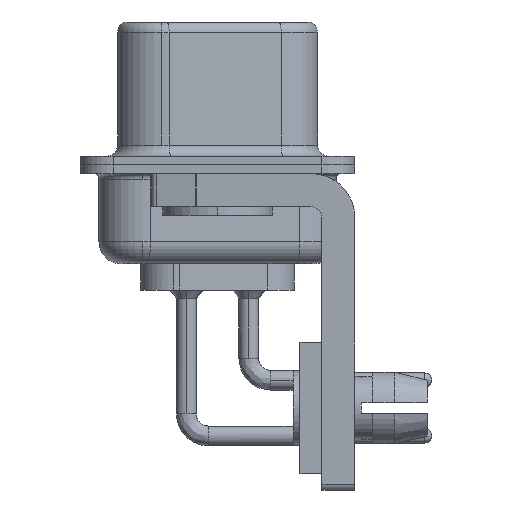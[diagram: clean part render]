
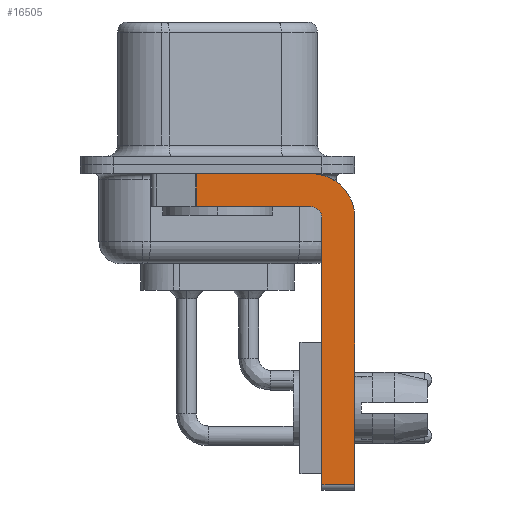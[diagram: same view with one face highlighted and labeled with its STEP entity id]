
A CAD part, left-side view. The second image highlights one B-rep face of the part: STEP entity #16505.
In plain terms, the highlighted planar face has unit normal (-1, 0, 0).
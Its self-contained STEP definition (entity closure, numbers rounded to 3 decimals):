
#245 = EDGE_CURVE ( 'NONE', #12847, #6155, #29911, .T. ) ;
#1064 = CARTESIAN_POINT ( 'NONE',  ( -2.9, -4.25, -2.4 ) ) ;
#1398 = DIRECTION ( 'NONE',  ( 1., 0., 0. ) ) ;
#1593 = ORIENTED_EDGE ( 'NONE', *, *, #245, .F. ) ;
#1625 = VECTOR ( 'NONE', #12792, 1000. ) ;
#1998 = LINE ( 'NONE', #26035, #20230 ) ;
#2313 = DIRECTION ( 'NONE',  ( 0., 0., -1. ) ) ;
#2340 = DIRECTION ( 'NONE',  ( 1., 0., 0. ) ) ;
#2969 = ORIENTED_EDGE ( 'NONE', *, *, #7836, .F. ) ;
#2994 = CARTESIAN_POINT ( 'NONE',  ( -2.9, 3., -0.4 ) ) ;
#3053 = CARTESIAN_POINT ( 'NONE',  ( -2.9, -4.75, -14.55 ) ) ;
#3404 = DIRECTION ( 'NONE',  ( 0., 0., 1. ) ) ;
#3484 = EDGE_LOOP ( 'NONE', ( #2969, #8541, #24831, #27332, #15916, #27538, #18704, #1593 ) ) ;
#3966 = VERTEX_POINT ( 'NONE', #19631 ) ;
#4508 = CARTESIAN_POINT ( 'NONE',  ( -2.9, -4.25, -1.9 ) ) ;
#4924 = VERTEX_POINT ( 'NONE', #22177 ) ;
#5443 = DIRECTION ( 'NONE',  ( 0., -1., 0. ) ) ;
#5707 = CARTESIAN_POINT ( 'NONE',  ( -2.9, 0.978, -1.9 ) ) ;
#6155 = VERTEX_POINT ( 'NONE', #12769 ) ;
#7708 = LINE ( 'NONE', #5707, #1625 ) ;
#7836 = EDGE_CURVE ( 'NONE', #9956, #12847, #29578, .T. ) ;
#7934 = EDGE_CURVE ( 'NONE', #3966, #4924, #8753, .T. ) ;
#8349 = CARTESIAN_POINT ( 'NONE',  ( -2.9, -4.25, -0.4 ) ) ;
#8541 = ORIENTED_EDGE ( 'NONE', *, *, #23324, .T. ) ;
#8753 = CIRCLE ( 'NONE', #9552, 0.5 ) ;
#9113 = DIRECTION ( 'NONE',  ( 0., 1., 0. ) ) ;
#9251 = DIRECTION ( 'NONE',  ( 0., 0., 1. ) ) ;
#9552 = AXIS2_PLACEMENT_3D ( 'NONE', #1064, #17651, #3404 ) ;
#9956 = VERTEX_POINT ( 'NONE', #14706 ) ;
#10140 = AXIS2_PLACEMENT_3D ( 'NONE', #15537, #1398, #17988 ) ;
#10215 = CARTESIAN_POINT ( 'NONE',  ( -2.9, -6.25, -14.55 ) ) ;
#10776 = VERTEX_POINT ( 'NONE', #10215 ) ;
#10847 = LINE ( 'NONE', #4508, #22965 ) ;
#11173 = CARTESIAN_POINT ( 'NONE',  ( -2.9, -6.25, -2.4 ) ) ;
#12101 = VECTOR ( 'NONE', #5443, 1000. ) ;
#12769 = CARTESIAN_POINT ( 'NONE',  ( -2.9, -6.25, -2.4 ) ) ;
#12792 = DIRECTION ( 'NONE',  ( 0., 0., -1. ) ) ;
#12847 = VERTEX_POINT ( 'NONE', #8349 ) ;
#13667 = VERTEX_POINT ( 'NONE', #3053 ) ;
#13710 = EDGE_CURVE ( 'NONE', #13667, #10776, #28885, .T. ) ;
#13992 = FACE_OUTER_BOUND ( 'NONE', #3484, .T. ) ;
#14706 = CARTESIAN_POINT ( 'NONE',  ( -2.9, 0.978, -0.4 ) ) ;
#14728 = DIRECTION ( 'NONE',  ( 0., -1., 0. ) ) ;
#15537 = CARTESIAN_POINT ( 'NONE',  ( -2.9, -4.25, -2.4 ) ) ;
#15916 = ORIENTED_EDGE ( 'NONE', *, *, #28440, .F. ) ;
#16208 = EDGE_CURVE ( 'NONE', #4924, #29342, #10847, .T. ) ;
#16505 = ADVANCED_FACE ( 'NONE', ( #13992 ), #24970, .F. ) ;
#16553 = AXIS2_PLACEMENT_3D ( 'NONE', #18113, #2340, #2313 ) ;
#16686 = EDGE_CURVE ( 'NONE', #6155, #10776, #28485, .T. ) ;
#17651 = DIRECTION ( 'NONE',  ( -1., 0., 0. ) ) ;
#17988 = DIRECTION ( 'NONE',  ( 0., 0., -1. ) ) ;
#18113 = CARTESIAN_POINT ( 'NONE',  ( -2.9, -4.25, -2.4 ) ) ;
#18704 = ORIENTED_EDGE ( 'NONE', *, *, #16686, .F. ) ;
#19631 = CARTESIAN_POINT ( 'NONE',  ( -2.9, -4.75, -2.4 ) ) ;
#19819 = CARTESIAN_POINT ( 'NONE',  ( -2.9, -4.25, -14.55 ) ) ;
#20230 = VECTOR ( 'NONE', #9251, 1000. ) ;
#20277 = CARTESIAN_POINT ( 'NONE',  ( -2.9, 0.978, -1.9 ) ) ;
#22177 = CARTESIAN_POINT ( 'NONE',  ( -2.9, -4.25, -1.9 ) ) ;
#22686 = VECTOR ( 'NONE', #14728, 1000. ) ;
#22965 = VECTOR ( 'NONE', #9113, 1000. ) ;
#23067 = VECTOR ( 'NONE', #27812, 1000. ) ;
#23324 = EDGE_CURVE ( 'NONE', #9956, #29342, #7708, .T. ) ;
#24831 = ORIENTED_EDGE ( 'NONE', *, *, #16208, .F. ) ;
#24970 = PLANE ( 'NONE',  #10140 ) ;
#26035 = CARTESIAN_POINT ( 'NONE',  ( -2.9, -4.75, -14.8 ) ) ;
#27332 = ORIENTED_EDGE ( 'NONE', *, *, #7934, .F. ) ;
#27538 = ORIENTED_EDGE ( 'NONE', *, *, #13710, .T. ) ;
#27812 = DIRECTION ( 'NONE',  ( 0., 0., -1. ) ) ;
#28440 = EDGE_CURVE ( 'NONE', #13667, #3966, #1998, .T. ) ;
#28485 = LINE ( 'NONE', #11173, #23067 ) ;
#28885 = LINE ( 'NONE', #19819, #12101 ) ;
#29342 = VERTEX_POINT ( 'NONE', #20277 ) ;
#29578 = LINE ( 'NONE', #2994, #22686 ) ;
#29911 = CIRCLE ( 'NONE', #16553, 2. ) ;
